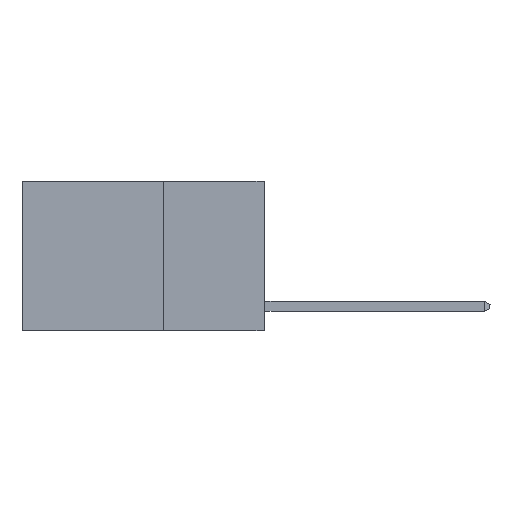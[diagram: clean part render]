
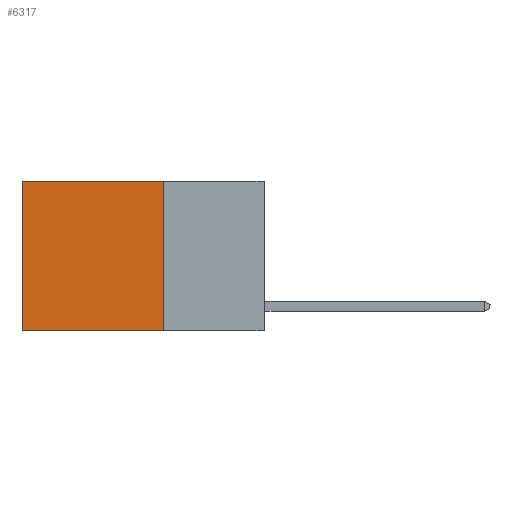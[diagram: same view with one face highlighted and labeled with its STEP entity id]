
A CAD part, left-side view. The second image highlights one B-rep face of the part: STEP entity #6317.
In plain terms, the highlighted planar face has unit normal (-1, 0, 0).
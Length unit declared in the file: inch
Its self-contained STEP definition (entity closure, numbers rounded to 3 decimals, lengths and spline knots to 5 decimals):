
#4 = CARTESIAN_POINT ( 'NONE',  ( 0.2625, 0.25, 0. ) ) ;
#152 = EDGE_CURVE ( 'NONE', #7072, #1621, #6639, .T. ) ;
#240 = DIRECTION ( 'NONE',  ( 0., 1., 0. ) ) ;
#801 = DIRECTION ( 'NONE',  ( 0., 0., -1. ) ) ;
#867 = VECTOR ( 'NONE', #6157, 39.37008 ) ;
#1180 = VECTOR ( 'NONE', #1513, 39.37008 ) ;
#1513 = DIRECTION ( 'NONE',  ( 0., 0., -1. ) ) ;
#1519 = LINE ( 'NONE', #8869, #1180 ) ;
#1571 = EDGE_LOOP ( 'NONE', ( #7744, #11612, #3464, #9815 ) ) ;
#1621 = VERTEX_POINT ( 'NONE', #5077 ) ;
#2022 = CARTESIAN_POINT ( 'NONE',  ( 0.2625, 0.25, 0. ) ) ;
#2171 = VECTOR ( 'NONE', #240, 39.37008 ) ;
#2496 = VERTEX_POINT ( 'NONE', #9039 ) ;
#3230 = CARTESIAN_POINT ( 'NONE',  ( 0.2625, 0.25, -0.37 ) ) ;
#3464 = ORIENTED_EDGE ( 'NONE', *, *, #12426, .F. ) ;
#3873 = CARTESIAN_POINT ( 'NONE',  ( 0.2625, 0.25, 0. ) ) ;
#4117 = EDGE_CURVE ( 'NONE', #2496, #1621, #1519, .T. ) ;
#4634 = DIRECTION ( 'NONE',  ( 1., 0., 0. ) ) ;
#5021 = CARTESIAN_POINT ( 'NONE',  ( 0.2625, 0.25, -0.37 ) ) ;
#5077 = CARTESIAN_POINT ( 'NONE',  ( 0.2625, 0.6, -0.37 ) ) ;
#5535 = LINE ( 'NONE', #2022, #2171 ) ;
#5588 = PLANE ( 'NONE',  #10863 ) ;
#5654 = VERTEX_POINT ( 'NONE', #4 ) ;
#5747 = FACE_OUTER_BOUND ( 'NONE', #1571, .T. ) ;
#6157 = DIRECTION ( 'NONE',  ( 0., 1., 0. ) ) ;
#6317 = ADVANCED_FACE ( 'NONE', ( #5747 ), #5588, .F. ) ;
#6639 = LINE ( 'NONE', #5021, #867 ) ;
#6641 = DIRECTION ( 'NONE',  ( 0., 0., -1. ) ) ;
#7072 = VERTEX_POINT ( 'NONE', #3230 ) ;
#7744 = ORIENTED_EDGE ( 'NONE', *, *, #4117, .T. ) ;
#8869 = CARTESIAN_POINT ( 'NONE',  ( 0.2625, 0.6, 0. ) ) ;
#9039 = CARTESIAN_POINT ( 'NONE',  ( 0.2625, 0.6, 0. ) ) ;
#9158 = VECTOR ( 'NONE', #801, 39.37008 ) ;
#9671 = EDGE_CURVE ( 'NONE', #5654, #2496, #5535, .T. ) ;
#9673 = CARTESIAN_POINT ( 'NONE',  ( 0.2625, 0.25, 0. ) ) ;
#9815 = ORIENTED_EDGE ( 'NONE', *, *, #9671, .T. ) ;
#10863 = AXIS2_PLACEMENT_3D ( 'NONE', #9673, #4634, #6641 ) ;
#11612 = ORIENTED_EDGE ( 'NONE', *, *, #152, .F. ) ;
#11833 = LINE ( 'NONE', #3873, #9158 ) ;
#12426 = EDGE_CURVE ( 'NONE', #5654, #7072, #11833, .T. ) ;
